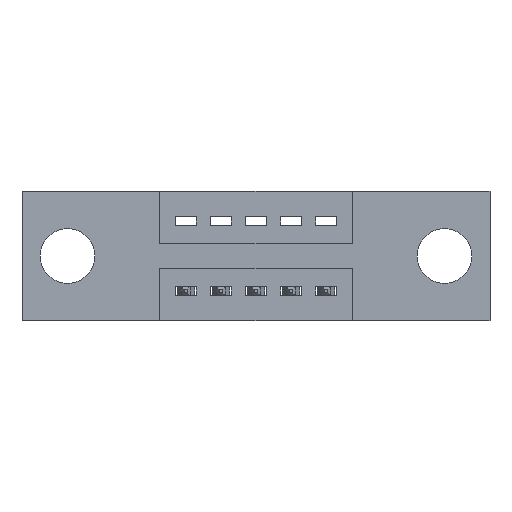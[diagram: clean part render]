
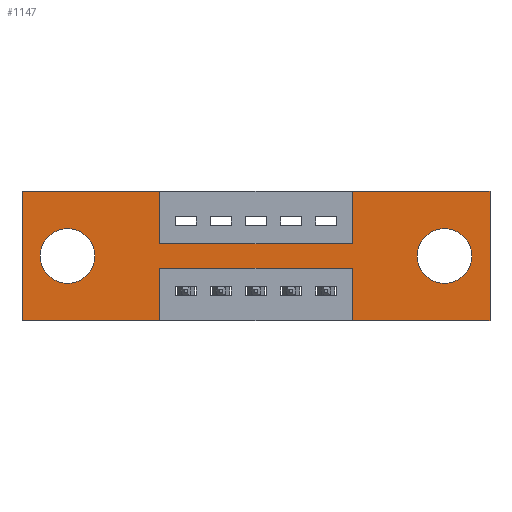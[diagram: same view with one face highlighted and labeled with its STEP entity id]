
A CAD part, front view. The second image highlights one B-rep face of the part: STEP entity #1147.
In plain terms, the highlighted planar face has unit normal (0, -1, 0).
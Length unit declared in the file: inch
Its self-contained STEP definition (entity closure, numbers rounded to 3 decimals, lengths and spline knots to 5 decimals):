
#182 = CARTESIAN_POINT ( 'NONE',  ( 0.3925, 0., -0.37 ) ) ;
#202 = ORIENTED_EDGE ( 'NONE', *, *, #8125, .F. ) ;
#247 = DIRECTION ( 'NONE',  ( 0., 0., 1. ) ) ;
#295 = CARTESIAN_POINT ( 'NONE',  ( 0.3925, 0., -0.22 ) ) ;
#342 = CARTESIAN_POINT ( 'NONE',  ( 0.13, 0., -0.263 ) ) ;
#391 = DIRECTION ( 'NONE',  ( 0., 0., -1. ) ) ;
#410 = CARTESIAN_POINT ( 'NONE',  ( 0., 0., -0.37 ) ) ;
#454 = CARTESIAN_POINT ( 'NONE',  ( 0.3925, 0., -0.15 ) ) ;
#468 = DIRECTION ( 'NONE',  ( 1., 0., 0. ) ) ;
#526 = VERTEX_POINT ( 'NONE', #2257 ) ;
#600 = FACE_OUTER_BOUND ( 'NONE', #4131, .T. ) ;
#647 = CARTESIAN_POINT ( 'NONE',  ( 1.335, 0., 0. ) ) ;
#702 = CIRCLE ( 'NONE', #1865, 0.078 ) ;
#732 = ORIENTED_EDGE ( 'NONE', *, *, #8506, .F. ) ;
#761 = CIRCLE ( 'NONE', #1213, 0.078 ) ;
#788 = CARTESIAN_POINT ( 'NONE',  ( 1.205, 0., -0.185 ) ) ;
#999 = LINE ( 'NONE', #5197, #2803 ) ;
#1100 = EDGE_CURVE ( 'NONE', #7754, #2493, #8446, .T. ) ;
#1142 = VERTEX_POINT ( 'NONE', #1673 ) ;
#1147 = ADVANCED_FACE ( 'NONE', ( #4731, #2917, #600 ), #3765, .T. ) ;
#1155 = EDGE_LOOP ( 'NONE', ( #4658, #8712 ) ) ;
#1181 = ORIENTED_EDGE ( 'NONE', *, *, #2015, .F. ) ;
#1213 = AXIS2_PLACEMENT_3D ( 'NONE', #7050, #5126, #7107 ) ;
#1288 = LINE ( 'NONE', #8482, #3422 ) ;
#1326 = EDGE_CURVE ( 'NONE', #8374, #6984, #1416, .T. ) ;
#1412 = ORIENTED_EDGE ( 'NONE', *, *, #1100, .T. ) ;
#1416 = LINE ( 'NONE', #3722, #6635 ) ;
#1475 = EDGE_CURVE ( 'NONE', #2493, #7754, #702, .T. ) ;
#1507 = VECTOR ( 'NONE', #4118, 39.37008 ) ;
#1606 = LINE ( 'NONE', #454, #8731 ) ;
#1673 = CARTESIAN_POINT ( 'NONE',  ( 0.9425, 0., -0.22 ) ) ;
#1821 = VERTEX_POINT ( 'NONE', #7002 ) ;
#1865 = AXIS2_PLACEMENT_3D ( 'NONE', #7478, #8159, #6138 ) ;
#1927 = EDGE_CURVE ( 'NONE', #3814, #8374, #999, .T. ) ;
#2007 = CARTESIAN_POINT ( 'NONE',  ( 0.3925, 0., -0.37 ) ) ;
#2015 = EDGE_CURVE ( 'NONE', #3467, #4629, #6309, .T. ) ;
#2245 = EDGE_CURVE ( 'NONE', #526, #1142, #4076, .T. ) ;
#2257 = CARTESIAN_POINT ( 'NONE',  ( 0.9425, 0., -0.37 ) ) ;
#2268 = CARTESIAN_POINT ( 'NONE',  ( 0., 0., 0. ) ) ;
#2493 = VERTEX_POINT ( 'NONE', #342 ) ;
#2620 = AXIS2_PLACEMENT_3D ( 'NONE', #410, #8501, #4366 ) ;
#2691 = ORIENTED_EDGE ( 'NONE', *, *, #7311, .F. ) ;
#2711 = DIRECTION ( 'NONE',  ( 0., 0., -1. ) ) ;
#2803 = VECTOR ( 'NONE', #468, 39.37008 ) ;
#2805 = DIRECTION ( 'NONE',  ( 0., 0., 1. ) ) ;
#2841 = ORIENTED_EDGE ( 'NONE', *, *, #2245, .F. ) ;
#2842 = DIRECTION ( 'NONE',  ( 0., 0., 1. ) ) ;
#2917 = FACE_BOUND ( 'NONE', #7594, .T. ) ;
#2989 = DIRECTION ( 'NONE',  ( -1., 0., 0. ) ) ;
#3052 = EDGE_CURVE ( 'NONE', #5733, #6994, #7038, .T. ) ;
#3192 = CARTESIAN_POINT ( 'NONE',  ( 0.9425, 0., -0.37 ) ) ;
#3422 = VECTOR ( 'NONE', #2842, 39.37008 ) ;
#3467 = VERTEX_POINT ( 'NONE', #182 ) ;
#3537 = ORIENTED_EDGE ( 'NONE', *, *, #8765, .F. ) ;
#3582 = CARTESIAN_POINT ( 'NONE',  ( 0.13, 0., -0.185 ) ) ;
#3718 = CARTESIAN_POINT ( 'NONE',  ( 0., 0., -0.37 ) ) ;
#3722 = CARTESIAN_POINT ( 'NONE',  ( 0.3925, 0., 0. ) ) ;
#3765 = PLANE ( 'NONE',  #2620 ) ;
#3814 = VERTEX_POINT ( 'NONE', #4436 ) ;
#3923 = ORIENTED_EDGE ( 'NONE', *, *, #6995, .F. ) ;
#4008 = AXIS2_PLACEMENT_3D ( 'NONE', #788, #4117, #2711 ) ;
#4076 = LINE ( 'NONE', #3192, #7369 ) ;
#4117 = DIRECTION ( 'NONE',  ( 0., 1., 0. ) ) ;
#4118 = DIRECTION ( 'NONE',  ( -1., 0., 0. ) ) ;
#4131 = EDGE_LOOP ( 'NONE', ( #732, #202, #2841, #3537, #6185, #5238, #2691, #3923, #7710, #7223, #5455, #1181 ) ) ;
#4149 = CARTESIAN_POINT ( 'NONE',  ( 0., 0., -0.37 ) ) ;
#4197 = CARTESIAN_POINT ( 'NONE',  ( 0., 0., -0.37 ) ) ;
#4342 = EDGE_CURVE ( 'NONE', #7974, #8493, #6679, .T. ) ;
#4366 = DIRECTION ( 'NONE',  ( 0., 0., -1. ) ) ;
#4436 = CARTESIAN_POINT ( 'NONE',  ( 0., 0., 0. ) ) ;
#4608 = DIRECTION ( 'NONE',  ( 1., 0., 0. ) ) ;
#4629 = VERTEX_POINT ( 'NONE', #4197 ) ;
#4653 = CARTESIAN_POINT ( 'NONE',  ( 0.3925, 0., 0. ) ) ;
#4658 = ORIENTED_EDGE ( 'NONE', *, *, #8684, .T. ) ;
#4731 = FACE_BOUND ( 'NONE', #1155, .T. ) ;
#4734 = DIRECTION ( 'NONE',  ( 0., 0., -1. ) ) ;
#5098 = DIRECTION ( 'NONE',  ( 0., 0., -1. ) ) ;
#5126 = DIRECTION ( 'NONE',  ( 0., 1., 0. ) ) ;
#5146 = CARTESIAN_POINT ( 'NONE',  ( 0.9425, 0., -0.15 ) ) ;
#5170 = EDGE_CURVE ( 'NONE', #8493, #1821, #5933, .T. ) ;
#5172 = VERTEX_POINT ( 'NONE', #5146 ) ;
#5187 = CARTESIAN_POINT ( 'NONE',  ( 1.205, 0., -0.107 ) ) ;
#5197 = CARTESIAN_POINT ( 'NONE',  ( 0., 0., 0. ) ) ;
#5238 = ORIENTED_EDGE ( 'NONE', *, *, #4342, .F. ) ;
#5314 = CARTESIAN_POINT ( 'NONE',  ( 0.3925, 0., -0.22 ) ) ;
#5454 = VECTOR ( 'NONE', #2805, 39.37008 ) ;
#5455 = ORIENTED_EDGE ( 'NONE', *, *, #7181, .F. ) ;
#5667 = LINE ( 'NONE', #8184, #5454 ) ;
#5733 = VERTEX_POINT ( 'NONE', #7807 ) ;
#5850 = VECTOR ( 'NONE', #7082, 39.37008 ) ;
#5922 = VECTOR ( 'NONE', #391, 39.37008 ) ;
#5933 = LINE ( 'NONE', #7921, #5922 ) ;
#5958 = LINE ( 'NONE', #3718, #5850 ) ;
#6138 = DIRECTION ( 'NONE',  ( 0., 0., 1. ) ) ;
#6185 = ORIENTED_EDGE ( 'NONE', *, *, #5170, .F. ) ;
#6309 = LINE ( 'NONE', #4149, #1507 ) ;
#6488 = AXIS2_PLACEMENT_3D ( 'NONE', #3582, #8396, #247 ) ;
#6635 = VECTOR ( 'NONE', #5098, 39.37008 ) ;
#6679 = LINE ( 'NONE', #2268, #6900 ) ;
#6900 = VECTOR ( 'NONE', #7794, 39.37008 ) ;
#6984 = VERTEX_POINT ( 'NONE', #7155 ) ;
#6994 = VERTEX_POINT ( 'NONE', #5187 ) ;
#6995 = EDGE_CURVE ( 'NONE', #6984, #5172, #1606, .T. ) ;
#7002 = CARTESIAN_POINT ( 'NONE',  ( 1.335, 0., -0.37 ) ) ;
#7014 = VECTOR ( 'NONE', #4734, 39.37008 ) ;
#7038 = CIRCLE ( 'NONE', #4008, 0.078 ) ;
#7050 = CARTESIAN_POINT ( 'NONE',  ( 1.205, 0., -0.185 ) ) ;
#7082 = DIRECTION ( 'NONE',  ( -1., 0., 0. ) ) ;
#7107 = DIRECTION ( 'NONE',  ( 0., 0., -1. ) ) ;
#7155 = CARTESIAN_POINT ( 'NONE',  ( 0.3925, 0., -0.15 ) ) ;
#7181 = EDGE_CURVE ( 'NONE', #4629, #3814, #1288, .T. ) ;
#7223 = ORIENTED_EDGE ( 'NONE', *, *, #1927, .F. ) ;
#7268 = DIRECTION ( 'NONE',  ( 0., 0., 1. ) ) ;
#7311 = EDGE_CURVE ( 'NONE', #5172, #7974, #5667, .T. ) ;
#7369 = VECTOR ( 'NONE', #7268, 39.37008 ) ;
#7478 = CARTESIAN_POINT ( 'NONE',  ( 0.13, 0., -0.185 ) ) ;
#7594 = EDGE_LOOP ( 'NONE', ( #1412, #7751 ) ) ;
#7614 = CARTESIAN_POINT ( 'NONE',  ( 0.9425, 0., 0. ) ) ;
#7710 = ORIENTED_EDGE ( 'NONE', *, *, #1326, .F. ) ;
#7751 = ORIENTED_EDGE ( 'NONE', *, *, #1475, .T. ) ;
#7754 = VERTEX_POINT ( 'NONE', #8664 ) ;
#7794 = DIRECTION ( 'NONE',  ( 1., 0., 0. ) ) ;
#7807 = CARTESIAN_POINT ( 'NONE',  ( 1.205, 0., -0.263 ) ) ;
#7921 = CARTESIAN_POINT ( 'NONE',  ( 1.335, 0., 0. ) ) ;
#7974 = VERTEX_POINT ( 'NONE', #7614 ) ;
#7999 = LINE ( 'NONE', #295, #8189 ) ;
#8125 = EDGE_CURVE ( 'NONE', #1142, #8312, #7999, .T. ) ;
#8159 = DIRECTION ( 'NONE',  ( 0., 1., 0. ) ) ;
#8184 = CARTESIAN_POINT ( 'NONE',  ( 0.9425, 0., 0. ) ) ;
#8189 = VECTOR ( 'NONE', #2989, 39.37008 ) ;
#8312 = VERTEX_POINT ( 'NONE', #5314 ) ;
#8374 = VERTEX_POINT ( 'NONE', #4653 ) ;
#8396 = DIRECTION ( 'NONE',  ( 0., 1., 0. ) ) ;
#8446 = CIRCLE ( 'NONE', #6488, 0.078 ) ;
#8482 = CARTESIAN_POINT ( 'NONE',  ( 0., 0., 0. ) ) ;
#8490 = LINE ( 'NONE', #2007, #7014 ) ;
#8493 = VERTEX_POINT ( 'NONE', #647 ) ;
#8501 = DIRECTION ( 'NONE',  ( 0., -1., 0. ) ) ;
#8506 = EDGE_CURVE ( 'NONE', #8312, #3467, #8490, .T. ) ;
#8664 = CARTESIAN_POINT ( 'NONE',  ( 0.13, 0., -0.107 ) ) ;
#8684 = EDGE_CURVE ( 'NONE', #6994, #5733, #761, .T. ) ;
#8712 = ORIENTED_EDGE ( 'NONE', *, *, #3052, .T. ) ;
#8731 = VECTOR ( 'NONE', #4608, 39.37008 ) ;
#8765 = EDGE_CURVE ( 'NONE', #1821, #526, #5958, .T. ) ;
